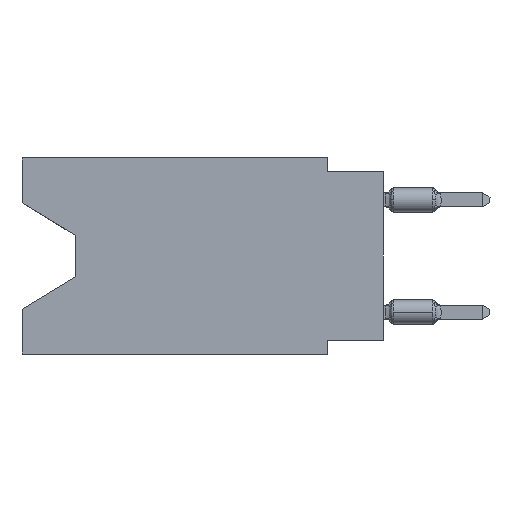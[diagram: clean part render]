
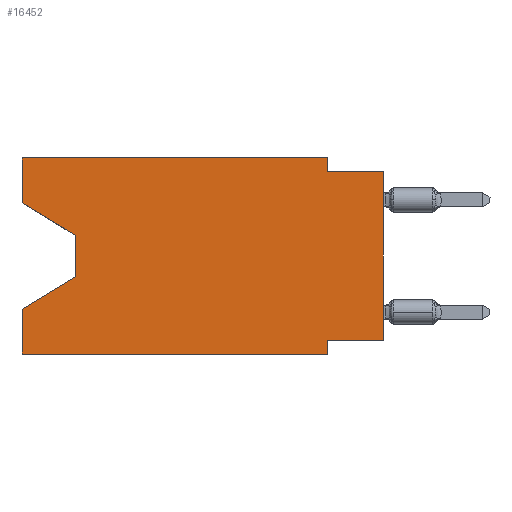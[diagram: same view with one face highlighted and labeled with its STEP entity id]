
A CAD part, left-side view. The second image highlights one B-rep face of the part: STEP entity #16452.
In plain terms, the highlighted planar face has unit normal (-1, 0, 0).
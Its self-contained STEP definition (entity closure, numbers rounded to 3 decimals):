
#121 = CARTESIAN_POINT ( 'NONE',  ( 0., 0., -0.635 ) ) ;
#258 = CARTESIAN_POINT ( 'NONE',  ( 0., 13.97, -3.505 ) ) ;
#327 = CARTESIAN_POINT ( 'NONE',  ( 0., 16.383, -8.89 ) ) ;
#347 = CARTESIAN_POINT ( 'NONE',  ( 0., 2.54, -0.635 ) ) ;
#721 = DIRECTION ( 'NONE',  ( 0., 0., 1. ) ) ;
#1157 = DIRECTION ( 'NONE',  ( 0., 0.855, -0.519 ) ) ;
#1753 = CARTESIAN_POINT ( 'NONE',  ( 0., 16.383, -2.038 ) ) ;
#2020 = CARTESIAN_POINT ( 'NONE',  ( 0., 0., 0. ) ) ;
#2225 = LINE ( 'NONE', #14539, #13514 ) ;
#2530 = LINE ( 'NONE', #15288, #21257 ) ;
#2892 = DIRECTION ( 'NONE',  ( 1., 0., 0. ) ) ;
#2967 = ORIENTED_EDGE ( 'NONE', *, *, #14806, .F. ) ;
#3427 = LINE ( 'NONE', #21070, #9799 ) ;
#3522 = VECTOR ( 'NONE', #14576, 1000. ) ;
#4301 = ORIENTED_EDGE ( 'NONE', *, *, #18410, .F. ) ;
#4499 = LINE ( 'NONE', #11549, #8338 ) ;
#5193 = LINE ( 'NONE', #18802, #6563 ) ;
#5325 = CARTESIAN_POINT ( 'NONE',  ( 0., 2.54, -8.89 ) ) ;
#5614 = ORIENTED_EDGE ( 'NONE', *, *, #22000, .T. ) ;
#5676 = CARTESIAN_POINT ( 'NONE',  ( 0., 16.383, -2.038 ) ) ;
#5774 = CARTESIAN_POINT ( 'NONE',  ( 0., 0., -8.255 ) ) ;
#5777 = DIRECTION ( 'NONE',  ( 0., -0.855, -0.519 ) ) ;
#6199 = EDGE_CURVE ( 'NONE', #13107, #20383, #22298, .T. ) ;
#6236 = FACE_OUTER_BOUND ( 'NONE', #17000, .T. ) ;
#6460 = CARTESIAN_POINT ( 'NONE',  ( 0., 16.383, 0. ) ) ;
#6563 = VECTOR ( 'NONE', #12233, 1000. ) ;
#6842 = VERTEX_POINT ( 'NONE', #10630 ) ;
#7250 = CARTESIAN_POINT ( 'NONE',  ( 0., 13.97, -5.385 ) ) ;
#7759 = VERTEX_POINT ( 'NONE', #5676 ) ;
#7835 = CARTESIAN_POINT ( 'NONE',  ( 0., 2.54, 0. ) ) ;
#8182 = LINE ( 'NONE', #7835, #14935 ) ;
#8204 = VECTOR ( 'NONE', #11486, 1000. ) ;
#8338 = VECTOR ( 'NONE', #1157, 1000. ) ;
#8354 = VERTEX_POINT ( 'NONE', #10145 ) ;
#8514 = DIRECTION ( 'NONE',  ( 0., 0., 1. ) ) ;
#8783 = EDGE_CURVE ( 'NONE', #20383, #18175, #2530, .T. ) ;
#9024 = LINE ( 'NONE', #18233, #12225 ) ;
#9082 = LINE ( 'NONE', #327, #19292 ) ;
#9228 = LINE ( 'NONE', #121, #16879 ) ;
#9799 = VECTOR ( 'NONE', #8514, 1000. ) ;
#9811 = PLANE ( 'NONE',  #17511 ) ;
#10145 = CARTESIAN_POINT ( 'NONE',  ( 0., 16.383, -8.89 ) ) ;
#10630 = CARTESIAN_POINT ( 'NONE',  ( 0., 0., -0.635 ) ) ;
#10662 = EDGE_CURVE ( 'NONE', #7759, #10723, #17529, .T. ) ;
#10723 = VERTEX_POINT ( 'NONE', #258 ) ;
#11464 = DIRECTION ( 'NONE',  ( 0., 0., -1. ) ) ;
#11486 = DIRECTION ( 'NONE',  ( 0., 1., 0. ) ) ;
#11549 = CARTESIAN_POINT ( 'NONE',  ( 0., 13.97, -5.385 ) ) ;
#11577 = ORIENTED_EDGE ( 'NONE', *, *, #18533, .F. ) ;
#11718 = CARTESIAN_POINT ( 'NONE',  ( 0., 0., -8.255 ) ) ;
#11930 = CARTESIAN_POINT ( 'NONE',  ( 0., 16.383, 0. ) ) ;
#12156 = ORIENTED_EDGE ( 'NONE', *, *, #10662, .T. ) ;
#12225 = VECTOR ( 'NONE', #11464, 1000. ) ;
#12233 = DIRECTION ( 'NONE',  ( 0., -1., 0. ) ) ;
#12380 = VERTEX_POINT ( 'NONE', #347 ) ;
#12463 = DIRECTION ( 'NONE',  ( 0., -1., 0. ) ) ;
#13000 = CARTESIAN_POINT ( 'NONE',  ( 0., 2.54, -8.255 ) ) ;
#13033 = ORIENTED_EDGE ( 'NONE', *, *, #21512, .T. ) ;
#13107 = VERTEX_POINT ( 'NONE', #5774 ) ;
#13322 = VERTEX_POINT ( 'NONE', #7250 ) ;
#13514 = VECTOR ( 'NONE', #721, 1000. ) ;
#13517 = VERTEX_POINT ( 'NONE', #20778 ) ;
#14426 = ORIENTED_EDGE ( 'NONE', *, *, #8783, .F. ) ;
#14539 = CARTESIAN_POINT ( 'NONE',  ( 0., 16.383, 0. ) ) ;
#14576 = DIRECTION ( 'NONE',  ( 0., 0., 1. ) ) ;
#14806 = EDGE_CURVE ( 'NONE', #8354, #15376, #2225, .T. ) ;
#14935 = VECTOR ( 'NONE', #16470, 1000. ) ;
#15288 = CARTESIAN_POINT ( 'NONE',  ( 0., 2.54, -8.89 ) ) ;
#15370 = EDGE_CURVE ( 'NONE', #13517, #12380, #8182, .T. ) ;
#15376 = VERTEX_POINT ( 'NONE', #18664 ) ;
#15465 = EDGE_CURVE ( 'NONE', #7759, #15757, #3427, .T. ) ;
#15757 = VERTEX_POINT ( 'NONE', #11930 ) ;
#15934 = ORIENTED_EDGE ( 'NONE', *, *, #15465, .F. ) ;
#16452 = ADVANCED_FACE ( 'NONE', ( #6236 ), #9811, .F. ) ;
#16470 = DIRECTION ( 'NONE',  ( 0., 0., -1. ) ) ;
#16488 = EDGE_CURVE ( 'NONE', #13322, #15376, #4499, .T. ) ;
#16879 = VECTOR ( 'NONE', #12463, 1000. ) ;
#17000 = EDGE_LOOP ( 'NONE', ( #12156, #5614, #18089, #2967, #21449, #14426, #22557, #13033, #11577, #20558, #4301, #15934 ) ) ;
#17511 = AXIS2_PLACEMENT_3D ( 'NONE', #6460, #2892, #22029 ) ;
#17529 = LINE ( 'NONE', #1753, #20791 ) ;
#17794 = LINE ( 'NONE', #2020, #3522 ) ;
#17821 = DIRECTION ( 'NONE',  ( 0., -1., 0. ) ) ;
#18089 = ORIENTED_EDGE ( 'NONE', *, *, #16488, .T. ) ;
#18175 = VERTEX_POINT ( 'NONE', #5325 ) ;
#18233 = CARTESIAN_POINT ( 'NONE',  ( 0., 13.97, -3.505 ) ) ;
#18410 = EDGE_CURVE ( 'NONE', #15757, #13517, #5193, .T. ) ;
#18533 = EDGE_CURVE ( 'NONE', #12380, #6842, #9228, .T. ) ;
#18664 = CARTESIAN_POINT ( 'NONE',  ( 0., 16.383, -6.852 ) ) ;
#18802 = CARTESIAN_POINT ( 'NONE',  ( 0., 16.383, 0. ) ) ;
#19057 = EDGE_CURVE ( 'NONE', #8354, #18175, #9082, .T. ) ;
#19292 = VECTOR ( 'NONE', #17821, 1000. ) ;
#20383 = VERTEX_POINT ( 'NONE', #13000 ) ;
#20558 = ORIENTED_EDGE ( 'NONE', *, *, #15370, .F. ) ;
#20778 = CARTESIAN_POINT ( 'NONE',  ( 0., 2.54, 0. ) ) ;
#20791 = VECTOR ( 'NONE', #5777, 1000. ) ;
#21070 = CARTESIAN_POINT ( 'NONE',  ( 0., 16.383, 0. ) ) ;
#21257 = VECTOR ( 'NONE', #22337, 1000. ) ;
#21449 = ORIENTED_EDGE ( 'NONE', *, *, #19057, .T. ) ;
#21512 = EDGE_CURVE ( 'NONE', #13107, #6842, #17794, .T. ) ;
#22000 = EDGE_CURVE ( 'NONE', #10723, #13322, #9024, .T. ) ;
#22029 = DIRECTION ( 'NONE',  ( 0., 0., -1. ) ) ;
#22298 = LINE ( 'NONE', #11718, #8204 ) ;
#22337 = DIRECTION ( 'NONE',  ( 0., 0., -1. ) ) ;
#22557 = ORIENTED_EDGE ( 'NONE', *, *, #6199, .F. ) ;
